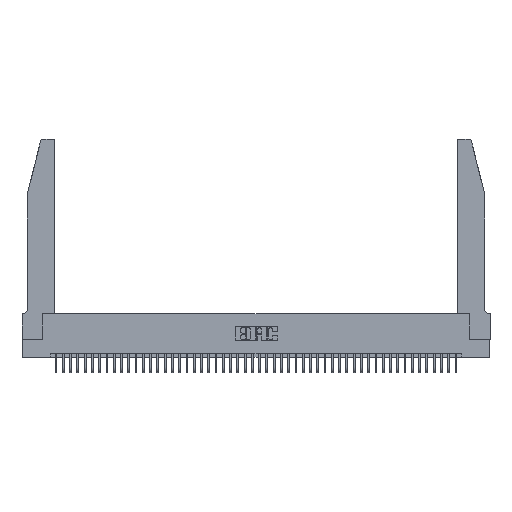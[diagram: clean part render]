
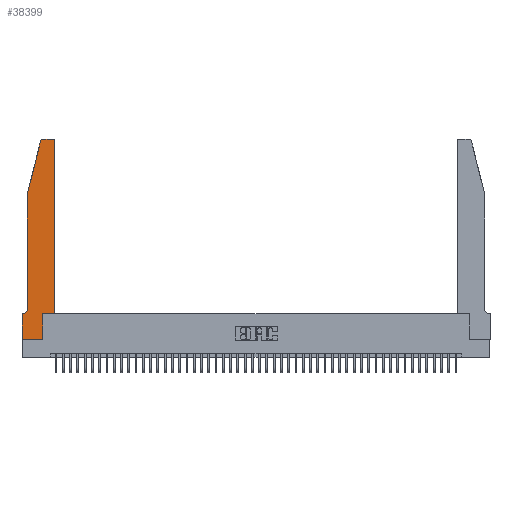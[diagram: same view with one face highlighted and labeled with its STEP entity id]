
A CAD part, top view. The second image highlights one B-rep face of the part: STEP entity #38399.
In plain terms, the highlighted planar face has unit normal (0, 0, 1).
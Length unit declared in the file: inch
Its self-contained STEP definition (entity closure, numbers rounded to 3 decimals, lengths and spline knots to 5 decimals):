
#213 = CIRCLE ( 'NONE', #45793, 0.03 ) ;
#818 = ORIENTED_EDGE ( 'NONE', *, *, #1919, .T. ) ;
#1771 = CARTESIAN_POINT ( 'NONE',  ( 0., 0., 0.37 ) ) ;
#1919 = EDGE_CURVE ( 'NONE', #3553, #18781, #17085, .T. ) ;
#2090 = ORIENTED_EDGE ( 'NONE', *, *, #17328, .T. ) ;
#2179 = CARTESIAN_POINT ( 'NONE',  ( 0.25487, 2.72718, 0.37 ) ) ;
#2458 = VECTOR ( 'NONE', #23129, 39.37008 ) ;
#3399 = EDGE_CURVE ( 'NONE', #18125, #19753, #32789, .T. ) ;
#3432 = DIRECTION ( 'NONE',  ( 1., 0., 0. ) ) ;
#3553 = VERTEX_POINT ( 'NONE', #20658 ) ;
#4622 = VECTOR ( 'NONE', #40702, 39.37008 ) ;
#5636 = DIRECTION ( 'NONE',  ( 0., -1., 0. ) ) ;
#8641 = CARTESIAN_POINT ( 'NONE',  ( 0., 0., 0.37 ) ) ;
#8649 = LINE ( 'NONE', #18123, #30189 ) ;
#8986 = EDGE_CURVE ( 'NONE', #39399, #33676, #11066, .T. ) ;
#9313 = CIRCLE ( 'NONE', #31736, 0.03 ) ;
#9951 = VERTEX_POINT ( 'NONE', #37003 ) ;
#11066 = LINE ( 'NONE', #25258, #4622 ) ;
#11931 = EDGE_CURVE ( 'NONE', #9951, #37665, #16040, .T. ) ;
#11980 = AXIS2_PLACEMENT_3D ( 'NONE', #32053, #39582, #20929 ) ;
#12546 = VECTOR ( 'NONE', #21857, 39.37008 ) ;
#12672 = ORIENTED_EDGE ( 'NONE', *, *, #15896, .T. ) ;
#13792 = CARTESIAN_POINT ( 'NONE',  ( 0.0055, 0.35, 0.37 ) ) ;
#14392 = DIRECTION ( 'NONE',  ( 0., 1., 0. ) ) ;
#14879 = CARTESIAN_POINT ( 'NONE',  ( 0.4205, 2.72, 0.37 ) ) ;
#15896 = EDGE_CURVE ( 'NONE', #37665, #3553, #9313, .T. ) ;
#16040 = LINE ( 'NONE', #44805, #12546 ) ;
#17009 = CARTESIAN_POINT ( 'NONE',  ( 0.284, 2.75, 0.37 ) ) ;
#17085 = LINE ( 'NONE', #25042, #21150 ) ;
#17328 = EDGE_CURVE ( 'NONE', #33676, #31900, #30183, .T. ) ;
#17827 = CARTESIAN_POINT ( 'NONE',  ( 0.0755, 0.42, 0.37 ) ) ;
#18123 = CARTESIAN_POINT ( 'NONE',  ( 0.2865, 0.35, 0.37 ) ) ;
#18125 = VERTEX_POINT ( 'NONE', #13792 ) ;
#18642 = ORIENTED_EDGE ( 'NONE', *, *, #11931, .T. ) ;
#18781 = VERTEX_POINT ( 'NONE', #17009 ) ;
#18894 = FACE_OUTER_BOUND ( 'NONE', #22320, .T. ) ;
#19753 = VERTEX_POINT ( 'NONE', #35461 ) ;
#20404 = EDGE_CURVE ( 'NONE', #21130, #28168, #35239, .T. ) ;
#20658 = CARTESIAN_POINT ( 'NONE',  ( 0.4205, 2.75, 0.37 ) ) ;
#20929 = DIRECTION ( 'NONE',  ( -1., 0., 0. ) ) ;
#21121 = DIRECTION ( 'NONE',  ( -1., 0., 0. ) ) ;
#21130 = VERTEX_POINT ( 'NONE', #31598 ) ;
#21150 = VECTOR ( 'NONE', #21121, 39.37008 ) ;
#21857 = DIRECTION ( 'NONE',  ( 0., 1., 0. ) ) ;
#22320 = EDGE_LOOP ( 'NONE', ( #818, #29611, #25070, #2090, #38454, #23633, #26860, #43747, #34818, #29572, #18642, #12672 ) ) ;
#22786 = LINE ( 'NONE', #28049, #32228 ) ;
#23129 = DIRECTION ( 'NONE',  ( 1., 0., 0. ) ) ;
#23633 = ORIENTED_EDGE ( 'NONE', *, *, #3399, .T. ) ;
#23755 = DIRECTION ( 'NONE',  ( -1., 0., 0. ) ) ;
#24200 = CARTESIAN_POINT ( 'NONE',  ( 0.0755, 2., 0.37 ) ) ;
#24223 = VECTOR ( 'NONE', #5636, 39.37008 ) ;
#24580 = DIRECTION ( 'NONE',  ( 1., 0., 0. ) ) ;
#25042 = CARTESIAN_POINT ( 'NONE',  ( 0.2605, 2.75, 0.37 ) ) ;
#25070 = ORIENTED_EDGE ( 'NONE', *, *, #8986, .T. ) ;
#25258 = CARTESIAN_POINT ( 'NONE',  ( 0.0755, 2., 0.37 ) ) ;
#25779 = CARTESIAN_POINT ( 'NONE',  ( 0.0755, 2., 0.37 ) ) ;
#26080 = EDGE_CURVE ( 'NONE', #31900, #18125, #36173, .T. ) ;
#26860 = ORIENTED_EDGE ( 'NONE', *, *, #41847, .T. ) ;
#27504 = CARTESIAN_POINT ( 'NONE',  ( 0., 0.35, 0.37 ) ) ;
#28049 = CARTESIAN_POINT ( 'NONE',  ( 0.4505, 0.35, 0.37 ) ) ;
#28168 = VERTEX_POINT ( 'NONE', #47123 ) ;
#28600 = CARTESIAN_POINT ( 'NONE',  ( 0.284, 2.72, 0.37 ) ) ;
#28639 = EDGE_CURVE ( 'NONE', #18781, #39399, #213, .T. ) ;
#29572 = ORIENTED_EDGE ( 'NONE', *, *, #43901, .T. ) ;
#29611 = ORIENTED_EDGE ( 'NONE', *, *, #28639, .T. ) ;
#30183 = LINE ( 'NONE', #24200, #33113 ) ;
#30189 = VECTOR ( 'NONE', #14392, 39.37008 ) ;
#30534 = VERTEX_POINT ( 'NONE', #32297 ) ;
#31409 = DIRECTION ( 'NONE',  ( 0., 0., 1. ) ) ;
#31598 = CARTESIAN_POINT ( 'NONE',  ( 0., 0., 0.37 ) ) ;
#31736 = AXIS2_PLACEMENT_3D ( 'NONE', #14879, #36820, #3432 ) ;
#31900 = VERTEX_POINT ( 'NONE', #17827 ) ;
#32053 = CARTESIAN_POINT ( 'NONE',  ( 0.0055, 0.42, 0.37 ) ) ;
#32228 = VECTOR ( 'NONE', #24580, 39.37008 ) ;
#32297 = CARTESIAN_POINT ( 'NONE',  ( 0.2865, 0.35, 0.37 ) ) ;
#32789 = LINE ( 'NONE', #35066, #39252 ) ;
#33044 = EDGE_CURVE ( 'NONE', #28168, #30534, #8649, .T. ) ;
#33113 = VECTOR ( 'NONE', #43085, 39.37008 ) ;
#33676 = VERTEX_POINT ( 'NONE', #25779 ) ;
#34818 = ORIENTED_EDGE ( 'NONE', *, *, #33044, .T. ) ;
#35066 = CARTESIAN_POINT ( 'NONE',  ( 0.0755, 0.35, 0.37 ) ) ;
#35239 = LINE ( 'NONE', #8641, #2458 ) ;
#35461 = CARTESIAN_POINT ( 'NONE',  ( 0., 0.35, 0.37 ) ) ;
#35680 = PLANE ( 'NONE',  #42347 ) ;
#36106 = DIRECTION ( 'NONE',  ( 0., 0., 1. ) ) ;
#36173 = CIRCLE ( 'NONE', #11980, 0.07 ) ;
#36820 = DIRECTION ( 'NONE',  ( 0., 0., 1. ) ) ;
#37003 = CARTESIAN_POINT ( 'NONE',  ( 0.4505, 0.35, 0.37 ) ) ;
#37157 = LINE ( 'NONE', #1771, #24223 ) ;
#37665 = VERTEX_POINT ( 'NONE', #41664 ) ;
#38399 = ADVANCED_FACE ( 'NONE', ( #18894 ), #35680, .T. ) ;
#38454 = ORIENTED_EDGE ( 'NONE', *, *, #26080, .T. ) ;
#38809 = DIRECTION ( 'NONE',  ( 1., 0., 0. ) ) ;
#39252 = VECTOR ( 'NONE', #23755, 39.37008 ) ;
#39399 = VERTEX_POINT ( 'NONE', #2179 ) ;
#39582 = DIRECTION ( 'NONE',  ( 0., 0., -1. ) ) ;
#40702 = DIRECTION ( 'NONE',  ( -0.239, -0.971, 0. ) ) ;
#41664 = CARTESIAN_POINT ( 'NONE',  ( 0.4505, 2.72, 0.37 ) ) ;
#41847 = EDGE_CURVE ( 'NONE', #19753, #21130, #37157, .T. ) ;
#42347 = AXIS2_PLACEMENT_3D ( 'NONE', #27504, #31409, #38809 ) ;
#43085 = DIRECTION ( 'NONE',  ( 0., -1., 0. ) ) ;
#43747 = ORIENTED_EDGE ( 'NONE', *, *, #20404, .T. ) ;
#43901 = EDGE_CURVE ( 'NONE', #30534, #9951, #22786, .T. ) ;
#44805 = CARTESIAN_POINT ( 'NONE',  ( 0.4505, 0.35, 0.37 ) ) ;
#45793 = AXIS2_PLACEMENT_3D ( 'NONE', #28600, #36106, #47432 ) ;
#47123 = CARTESIAN_POINT ( 'NONE',  ( 0.2865, 0., 0.37 ) ) ;
#47432 = DIRECTION ( 'NONE',  ( 1., 0., 0. ) ) ;
